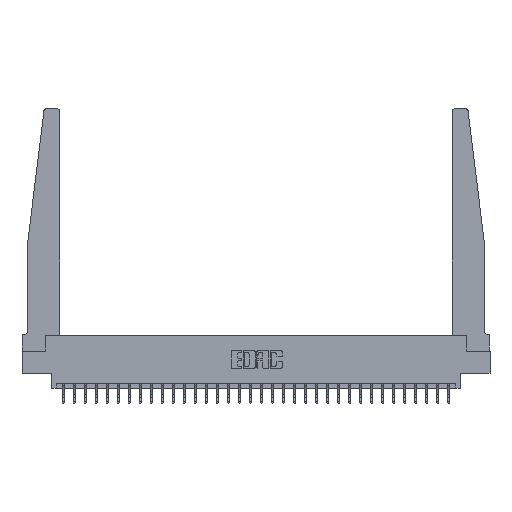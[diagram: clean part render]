
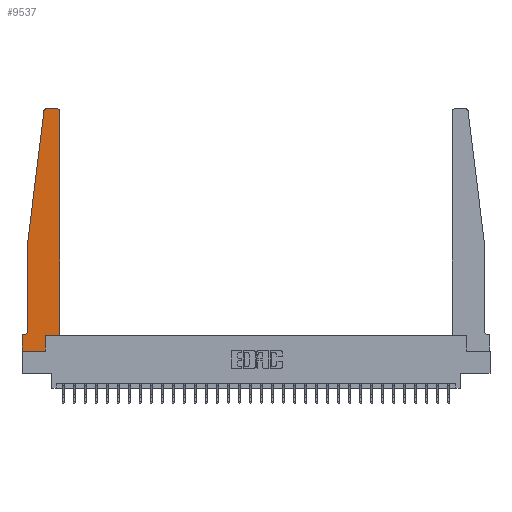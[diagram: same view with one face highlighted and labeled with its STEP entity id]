
A CAD part, top view. The second image highlights one B-rep face of the part: STEP entity #9537.
In plain terms, the highlighted planar face has unit normal (0, 0, 1).
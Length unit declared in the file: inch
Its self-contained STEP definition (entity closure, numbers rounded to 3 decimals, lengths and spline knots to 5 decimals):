
#2090 = EDGE_CURVE ( 'NONE', #27250, #5365, #21260, .T. ) ;
#2093 = CARTESIAN_POINT ( 'NONE',  ( 0.27653, 2.75, 0.37 ) ) ;
#2444 = VERTEX_POINT ( 'NONE', #28007 ) ;
#2494 = DIRECTION ( 'NONE',  ( 0., -1., 0. ) ) ;
#2703 = ORIENTED_EDGE ( 'NONE', *, *, #13617, .T. ) ;
#3272 = CARTESIAN_POINT ( 'NONE',  ( 0.065, 0.1875, 0.37 ) ) ;
#3450 = VERTEX_POINT ( 'NONE', #9048 ) ;
#3522 = EDGE_CURVE ( 'NONE', #2444, #27250, #26484, .T. ) ;
#4476 = EDGE_CURVE ( 'NONE', #21774, #4577, #24996, .T. ) ;
#4523 = LINE ( 'NONE', #7285, #27980 ) ;
#4577 = VERTEX_POINT ( 'NONE', #25522 ) ;
#4791 = ORIENTED_EDGE ( 'NONE', *, *, #24221, .T. ) ;
#4955 = VECTOR ( 'NONE', #13381, 39.37008 ) ;
#5037 = VERTEX_POINT ( 'NONE', #27380 ) ;
#5151 = CARTESIAN_POINT ( 'NONE',  ( 0.395, 2.72, 0.37 ) ) ;
#5365 = VERTEX_POINT ( 'NONE', #5919 ) ;
#5624 = CARTESIAN_POINT ( 'NONE',  ( 0.425, 0.18, 0.37 ) ) ;
#5919 = CARTESIAN_POINT ( 'NONE',  ( 0.015, 0.1875, 0.37 ) ) ;
#6418 = ORIENTED_EDGE ( 'NONE', *, *, #2090, .T. ) ;
#6842 = ORIENTED_EDGE ( 'NONE', *, *, #24104, .T. ) ;
#6921 = ORIENTED_EDGE ( 'NONE', *, *, #10087, .T. ) ;
#7285 = CARTESIAN_POINT ( 'NONE',  ( 0.2605, 0.18, 0.37 ) ) ;
#7488 = DIRECTION ( 'NONE',  ( 1., 0., 0. ) ) ;
#7941 = DIRECTION ( 'NONE',  ( 0., 1., 0. ) ) ;
#8129 = VECTOR ( 'NONE', #27329, 39.37008 ) ;
#8570 = AXIS2_PLACEMENT_3D ( 'NONE', #12830, #28640, #15127 ) ;
#9011 = CIRCLE ( 'NONE', #8570, 0.03 ) ;
#9048 = CARTESIAN_POINT ( 'NONE',  ( 0.24675, 2.72367, 0.37 ) ) ;
#9076 = VECTOR ( 'NONE', #22981, 39.37008 ) ;
#9206 = EDGE_LOOP ( 'NONE', ( #6842, #15168, #27120, #9778, #6418, #2703, #24889, #15481, #4791, #6921, #19817, #12512 ) ) ;
#9537 = ADVANCED_FACE ( 'NONE', ( #12149 ), #23971, .T. ) ;
#9778 = ORIENTED_EDGE ( 'NONE', *, *, #3522, .T. ) ;
#9897 = CIRCLE ( 'NONE', #16103, 0.03 ) ;
#10087 = EDGE_CURVE ( 'NONE', #11070, #5037, #28772, .T. ) ;
#10387 = DIRECTION ( 'NONE',  ( 0., 0., 1. ) ) ;
#10572 = VECTOR ( 'NONE', #7941, 39.37008 ) ;
#10641 = CARTESIAN_POINT ( 'NONE',  ( 0., 0.1875, 0.37 ) ) ;
#11070 = VERTEX_POINT ( 'NONE', #27533 ) ;
#11553 = LINE ( 'NONE', #3272, #12272 ) ;
#11625 = CARTESIAN_POINT ( 'NONE',  ( 0.065, 1.25, 0.37 ) ) ;
#12149 = FACE_OUTER_BOUND ( 'NONE', #9206, .T. ) ;
#12272 = VECTOR ( 'NONE', #21494, 39.37008 ) ;
#12512 = ORIENTED_EDGE ( 'NONE', *, *, #24254, .T. ) ;
#12830 = CARTESIAN_POINT ( 'NONE',  ( 0.27653, 2.72, 0.37 ) ) ;
#13120 = CARTESIAN_POINT ( 'NONE',  ( 0.015, 0.2375, 0.37 ) ) ;
#13381 = DIRECTION ( 'NONE',  ( 1., 0., 0. ) ) ;
#13617 = EDGE_CURVE ( 'NONE', #5365, #21774, #11553, .T. ) ;
#13793 = VERTEX_POINT ( 'NONE', #15400 ) ;
#14922 = LINE ( 'NONE', #25050, #8129 ) ;
#15127 = DIRECTION ( 'NONE',  ( 1., 0., 0. ) ) ;
#15167 = LINE ( 'NONE', #18441, #9076 ) ;
#15168 = ORIENTED_EDGE ( 'NONE', *, *, #28360, .T. ) ;
#15350 = CARTESIAN_POINT ( 'NONE',  ( 0.065, 0.2375, 0.37 ) ) ;
#15400 = CARTESIAN_POINT ( 'NONE',  ( 0.395, 2.75, 0.37 ) ) ;
#15423 = DIRECTION ( 'NONE',  ( -1., 0., 0. ) ) ;
#15481 = ORIENTED_EDGE ( 'NONE', *, *, #15898, .T. ) ;
#15898 = EDGE_CURVE ( 'NONE', #4577, #28161, #29164, .T. ) ;
#16103 = AXIS2_PLACEMENT_3D ( 'NONE', #5151, #21097, #7488 ) ;
#16467 = DIRECTION ( 'NONE',  ( 0., 1., 0. ) ) ;
#16746 = VECTOR ( 'NONE', #26511, 39.37008 ) ;
#18261 = EDGE_CURVE ( 'NONE', #5037, #20187, #28636, .T. ) ;
#18441 = CARTESIAN_POINT ( 'NONE',  ( 0.065, 1.25, 0.37 ) ) ;
#18534 = DIRECTION ( 'NONE',  ( 0., -1., 0. ) ) ;
#18992 = VECTOR ( 'NONE', #18534, 39.37008 ) ;
#19817 = ORIENTED_EDGE ( 'NONE', *, *, #18261, .T. ) ;
#20046 = EDGE_CURVE ( 'NONE', #3450, #2444, #15167, .T. ) ;
#20187 = VERTEX_POINT ( 'NONE', #21475 ) ;
#20476 = VECTOR ( 'NONE', #2494, 39.37008 ) ;
#21097 = DIRECTION ( 'NONE',  ( 0., 0., 1. ) ) ;
#21260 = CIRCLE ( 'NONE', #28144, 0.05 ) ;
#21475 = CARTESIAN_POINT ( 'NONE',  ( 0.425, 2.72, 0.37 ) ) ;
#21494 = DIRECTION ( 'NONE',  ( -1., 0., 0. ) ) ;
#21699 = CARTESIAN_POINT ( 'NONE',  ( 0., 0.1875, 0.37 ) ) ;
#21774 = VERTEX_POINT ( 'NONE', #10641 ) ;
#21941 = VERTEX_POINT ( 'NONE', #2093 ) ;
#22981 = DIRECTION ( 'NONE',  ( -0.122, -0.992, 0. ) ) ;
#23318 = CARTESIAN_POINT ( 'NONE',  ( 0.2605, 0., 0.37 ) ) ;
#23971 = PLANE ( 'NONE',  #28740 ) ;
#24104 = EDGE_CURVE ( 'NONE', #13793, #21941, #14922, .T. ) ;
#24221 = EDGE_CURVE ( 'NONE', #28161, #11070, #4523, .T. ) ;
#24254 = EDGE_CURVE ( 'NONE', #20187, #13793, #9897, .T. ) ;
#24257 = CARTESIAN_POINT ( 'NONE',  ( 0.425, 0.18, 0.37 ) ) ;
#24889 = ORIENTED_EDGE ( 'NONE', *, *, #4476, .T. ) ;
#24996 = LINE ( 'NONE', #27508, #18992 ) ;
#25050 = CARTESIAN_POINT ( 'NONE',  ( 0.25, 2.75, 0.37 ) ) ;
#25522 = CARTESIAN_POINT ( 'NONE',  ( 0., 0., 0.37 ) ) ;
#26230 = DIRECTION ( 'NONE',  ( 1., 0., 0. ) ) ;
#26484 = LINE ( 'NONE', #11625, #20476 ) ;
#26511 = DIRECTION ( 'NONE',  ( 1., 0., 0. ) ) ;
#26919 = CARTESIAN_POINT ( 'NONE',  ( 0., 0., 0.37 ) ) ;
#27120 = ORIENTED_EDGE ( 'NONE', *, *, #20046, .T. ) ;
#27250 = VERTEX_POINT ( 'NONE', #15350 ) ;
#27329 = DIRECTION ( 'NONE',  ( -1., 0., 0. ) ) ;
#27380 = CARTESIAN_POINT ( 'NONE',  ( 0.425, 0.18, 0.37 ) ) ;
#27508 = CARTESIAN_POINT ( 'NONE',  ( 0., 0., 0.37 ) ) ;
#27533 = CARTESIAN_POINT ( 'NONE',  ( 0.2605, 0.18, 0.37 ) ) ;
#27980 = VECTOR ( 'NONE', #16467, 39.37008 ) ;
#28007 = CARTESIAN_POINT ( 'NONE',  ( 0.065, 1.25, 0.37 ) ) ;
#28144 = AXIS2_PLACEMENT_3D ( 'NONE', #13120, #28941, #15423 ) ;
#28161 = VERTEX_POINT ( 'NONE', #23318 ) ;
#28360 = EDGE_CURVE ( 'NONE', #21941, #3450, #9011, .T. ) ;
#28636 = LINE ( 'NONE', #5624, #10572 ) ;
#28640 = DIRECTION ( 'NONE',  ( 0., 0., 1. ) ) ;
#28740 = AXIS2_PLACEMENT_3D ( 'NONE', #21699, #10387, #26230 ) ;
#28772 = LINE ( 'NONE', #24257, #16746 ) ;
#28941 = DIRECTION ( 'NONE',  ( 0., 0., -1. ) ) ;
#29164 = LINE ( 'NONE', #26919, #4955 ) ;
